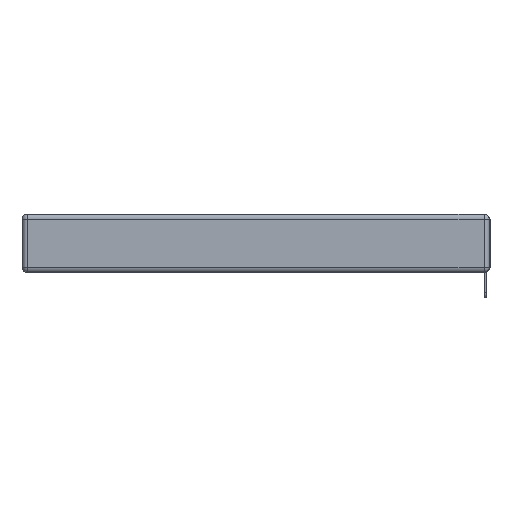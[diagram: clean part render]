
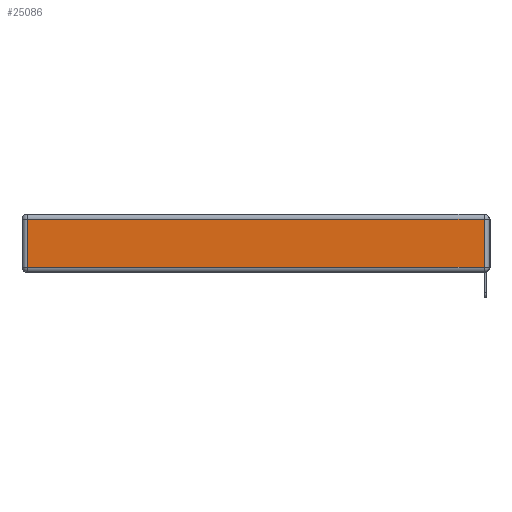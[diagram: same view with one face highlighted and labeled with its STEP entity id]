
A CAD part, left-side view. The second image highlights one B-rep face of the part: STEP entity #25086.
In plain terms, the highlighted planar face has unit normal (-1, 0, 0).
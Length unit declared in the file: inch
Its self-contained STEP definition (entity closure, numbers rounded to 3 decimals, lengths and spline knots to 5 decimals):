
#87 = VERTEX_POINT ( 'NONE', #18831 ) ;
#330 = VECTOR ( 'NONE', #20034, 39.37008 ) ;
#663 = CARTESIAN_POINT ( 'NONE',  ( 0., 2.72, -0.313 ) ) ;
#1023 = ORIENTED_EDGE ( 'NONE', *, *, #10561, .T. ) ;
#1677 = DIRECTION ( 'NONE',  ( -1., 0., 0. ) ) ;
#3362 = VERTEX_POINT ( 'NONE', #18788 ) ;
#3375 = VECTOR ( 'NONE', #18946, 39.37008 ) ;
#4625 = LINE ( 'NONE', #8871, #3375 ) ;
#5332 = EDGE_CURVE ( 'NONE', #20897, #20992, #19236, .T. ) ;
#5516 = CARTESIAN_POINT ( 'NONE',  ( 0., 0., -0.343 ) ) ;
#5706 = CARTESIAN_POINT ( 'NONE',  ( 0., 2.72, -0.343 ) ) ;
#5835 = DIRECTION ( 'NONE',  ( 0., 1., 0. ) ) ;
#6440 = DIRECTION ( 'NONE',  ( 0., 0., 1. ) ) ;
#7137 = VECTOR ( 'NONE', #5835, 39.37008 ) ;
#7577 = VECTOR ( 'NONE', #6440, 39.37008 ) ;
#7628 = ORIENTED_EDGE ( 'NONE', *, *, #5332, .T. ) ;
#7736 = PLANE ( 'NONE',  #16092 ) ;
#7779 = CARTESIAN_POINT ( 'NONE',  ( 0., 2.75, -0.03 ) ) ;
#8279 = CARTESIAN_POINT ( 'NONE',  ( 0., 2.72, -0.03 ) ) ;
#8640 = EDGE_CURVE ( 'NONE', #3362, #87, #23219, .T. ) ;
#8871 = CARTESIAN_POINT ( 'NONE',  ( 0., 0., -0.313 ) ) ;
#10374 = FACE_OUTER_BOUND ( 'NONE', #13136, .T. ) ;
#10561 = EDGE_CURVE ( 'NONE', #87, #20897, #13909, .T. ) ;
#13136 = EDGE_LOOP ( 'NONE', ( #25904, #17071, #1023, #7628 ) ) ;
#13655 = DIRECTION ( 'NONE',  ( 0., 0., 1. ) ) ;
#13909 = LINE ( 'NONE', #7779, #7137 ) ;
#16092 = AXIS2_PLACEMENT_3D ( 'NONE', #5516, #1677, #13655 ) ;
#16859 = CARTESIAN_POINT ( 'NONE',  ( 0., 0.03, -0.343 ) ) ;
#17071 = ORIENTED_EDGE ( 'NONE', *, *, #8640, .T. ) ;
#18788 = CARTESIAN_POINT ( 'NONE',  ( 0., 0.03, -0.313 ) ) ;
#18831 = CARTESIAN_POINT ( 'NONE',  ( 0., 0.03, -0.03 ) ) ;
#18946 = DIRECTION ( 'NONE',  ( 0., -1., 0. ) ) ;
#19209 = EDGE_CURVE ( 'NONE', #20992, #3362, #4625, .T. ) ;
#19236 = LINE ( 'NONE', #5706, #330 ) ;
#20034 = DIRECTION ( 'NONE',  ( 0., 0., -1. ) ) ;
#20897 = VERTEX_POINT ( 'NONE', #8279 ) ;
#20992 = VERTEX_POINT ( 'NONE', #663 ) ;
#23219 = LINE ( 'NONE', #16859, #7577 ) ;
#25086 = ADVANCED_FACE ( 'NONE', ( #10374 ), #7736, .T. ) ;
#25904 = ORIENTED_EDGE ( 'NONE', *, *, #19209, .T. ) ;
